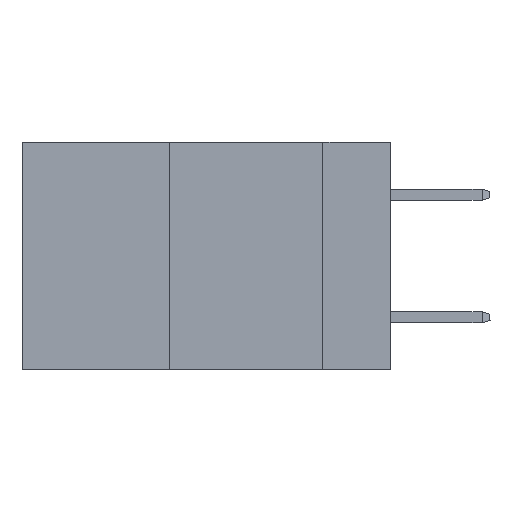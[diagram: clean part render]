
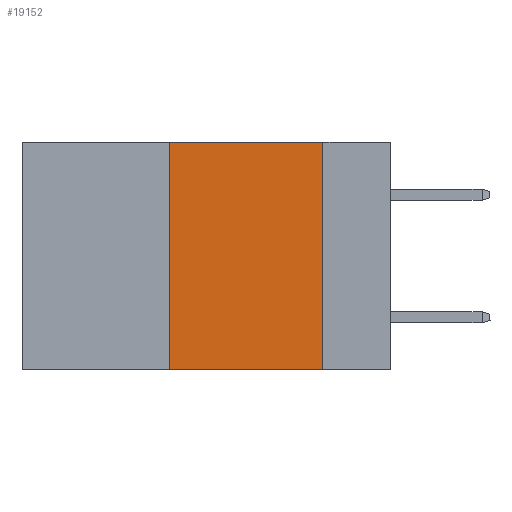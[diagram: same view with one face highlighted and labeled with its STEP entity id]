
A CAD part, left-side view. The second image highlights one B-rep face of the part: STEP entity #19152.
In plain terms, the highlighted planar face has unit normal (-1, 0, 0).
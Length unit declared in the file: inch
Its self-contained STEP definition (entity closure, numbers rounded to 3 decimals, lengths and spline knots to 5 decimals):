
#633 = LINE ( 'NONE', #30270, #3475 ) ;
#1745 = ORIENTED_EDGE ( 'NONE', *, *, #20766, .T. ) ;
#3178 = CARTESIAN_POINT ( 'NONE',  ( 0., 0.6, 0. ) ) ;
#3375 = CARTESIAN_POINT ( 'NONE',  ( 0., 0.36, 0. ) ) ;
#3475 = VECTOR ( 'NONE', #16876, 39.37008 ) ;
#3721 = VERTEX_POINT ( 'NONE', #39505 ) ;
#5055 = EDGE_LOOP ( 'NONE', ( #10756, #26180, #19948, #1745 ) ) ;
#6210 = DIRECTION ( 'NONE',  ( 1., 0., 0. ) ) ;
#6428 = FACE_OUTER_BOUND ( 'NONE', #5055, .T. ) ;
#9624 = EDGE_CURVE ( 'NONE', #21406, #41775, #38781, .T. ) ;
#9811 = LINE ( 'NONE', #23442, #10955 ) ;
#9957 = AXIS2_PLACEMENT_3D ( 'NONE', #3178, #6210, #25916 ) ;
#10756 = ORIENTED_EDGE ( 'NONE', *, *, #31222, .F. ) ;
#10955 = VECTOR ( 'NONE', #13053, 39.37008 ) ;
#11413 = EDGE_CURVE ( 'NONE', #22813, #21406, #633, .T. ) ;
#12794 = VECTOR ( 'NONE', #24388, 39.37008 ) ;
#13053 = DIRECTION ( 'NONE',  ( 0., 0., -1. ) ) ;
#14007 = LINE ( 'NONE', #27192, #12794 ) ;
#16519 = VECTOR ( 'NONE', #29250, 39.37008 ) ;
#16876 = DIRECTION ( 'NONE',  ( 0., 0., 1. ) ) ;
#19095 = CARTESIAN_POINT ( 'NONE',  ( 0., 0.6, 0. ) ) ;
#19152 = ADVANCED_FACE ( 'NONE', ( #6428 ), #19629, .F. ) ;
#19629 = PLANE ( 'NONE',  #9957 ) ;
#19762 = CARTESIAN_POINT ( 'NONE',  ( 0., 0.11, 0. ) ) ;
#19948 = ORIENTED_EDGE ( 'NONE', *, *, #11413, .F. ) ;
#20766 = EDGE_CURVE ( 'NONE', #22813, #3721, #14007, .T. ) ;
#21406 = VERTEX_POINT ( 'NONE', #3375 ) ;
#22813 = VERTEX_POINT ( 'NONE', #33665 ) ;
#23442 = CARTESIAN_POINT ( 'NONE',  ( 0., 0.11, 0. ) ) ;
#24388 = DIRECTION ( 'NONE',  ( 0., -1., 0. ) ) ;
#25916 = DIRECTION ( 'NONE',  ( 0., 0., -1. ) ) ;
#26180 = ORIENTED_EDGE ( 'NONE', *, *, #9624, .F. ) ;
#27192 = CARTESIAN_POINT ( 'NONE',  ( 0., 0.6, -0.37 ) ) ;
#29250 = DIRECTION ( 'NONE',  ( 0., -1., 0. ) ) ;
#30270 = CARTESIAN_POINT ( 'NONE',  ( 0., 0.36, 0. ) ) ;
#31222 = EDGE_CURVE ( 'NONE', #41775, #3721, #9811, .T. ) ;
#33665 = CARTESIAN_POINT ( 'NONE',  ( 0., 0.36, -0.37 ) ) ;
#38781 = LINE ( 'NONE', #19095, #16519 ) ;
#39505 = CARTESIAN_POINT ( 'NONE',  ( 0., 0.11, -0.37 ) ) ;
#41775 = VERTEX_POINT ( 'NONE', #19762 ) ;
